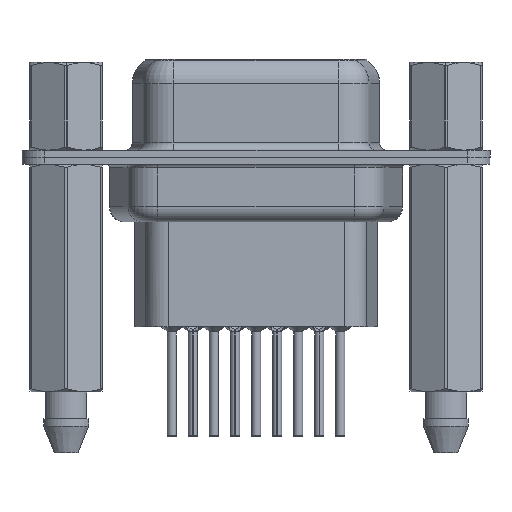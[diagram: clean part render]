
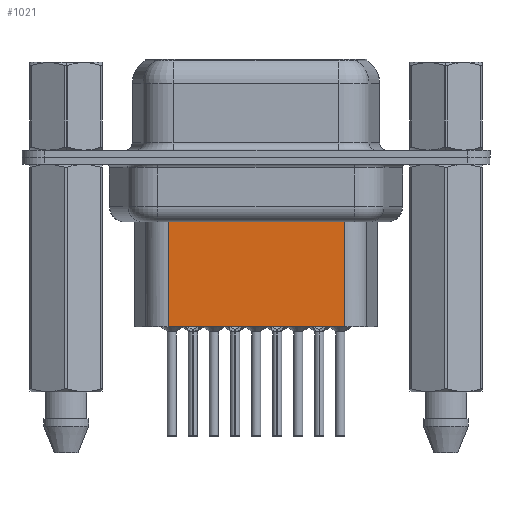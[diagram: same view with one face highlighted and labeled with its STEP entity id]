
A CAD part, front view. The second image highlights one B-rep face of the part: STEP entity #1021.
In plain terms, the highlighted planar face has unit normal (0, -1, 0).
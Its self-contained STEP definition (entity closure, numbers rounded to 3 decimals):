
#703 = ORIENTED_EDGE ( 'NONE', *, *, #12172, .T. ) ;
#1021 = ADVANCED_FACE ( 'NONE', ( #27451 ), #8354, .T. ) ;
#1368 = LINE ( 'NONE', #9865, #4313 ) ;
#1404 = DIRECTION ( 'NONE',  ( 1., 0., 0. ) ) ;
#1757 = DIRECTION ( 'NONE',  ( 0., 0., -1. ) ) ;
#2477 = CARTESIAN_POINT ( 'NONE',  ( 6.706, -3.5, -11.15 ) ) ;
#4313 = VECTOR ( 'NONE', #18347, 1000. ) ;
#4630 = VERTEX_POINT ( 'NONE', #13795 ) ;
#5192 = EDGE_CURVE ( 'NONE', #8631, #26141, #1368, .T. ) ;
#5831 = CARTESIAN_POINT ( 'NONE',  ( 6.706, -3.5, -3.1 ) ) ;
#6327 = EDGE_CURVE ( 'NONE', #8631, #4630, #18413, .T. ) ;
#6532 = VECTOR ( 'NONE', #9931, 1000. ) ;
#7393 = CARTESIAN_POINT ( 'NONE',  ( 18.294, -3.5, -11.15 ) ) ;
#8354 = PLANE ( 'NONE',  #12449 ) ;
#8631 = VERTEX_POINT ( 'NONE', #11443 ) ;
#9865 = CARTESIAN_POINT ( 'NONE',  ( 18.294, -3.5, -3.1 ) ) ;
#9931 = DIRECTION ( 'NONE',  ( -1., 0., 0. ) ) ;
#11034 = ORIENTED_EDGE ( 'NONE', *, *, #6327, .T. ) ;
#11443 = CARTESIAN_POINT ( 'NONE',  ( 18.294, -3.5, -4.097 ) ) ;
#11980 = VERTEX_POINT ( 'NONE', #21145 ) ;
#12172 = EDGE_CURVE ( 'NONE', #4630, #11980, #12220, .T. ) ;
#12220 = LINE ( 'NONE', #20705, #16073 ) ;
#12269 = ORIENTED_EDGE ( 'NONE', *, *, #21077, .F. ) ;
#12449 = AXIS2_PLACEMENT_3D ( 'NONE', #5831, #14080, #1404 ) ;
#13795 = CARTESIAN_POINT ( 'NONE',  ( 6.706, -3.5, -4.097 ) ) ;
#14080 = DIRECTION ( 'NONE',  ( 0., -1., 0. ) ) ;
#16073 = VECTOR ( 'NONE', #1757, 1000. ) ;
#18347 = DIRECTION ( 'NONE',  ( 0., 0., -1. ) ) ;
#18413 = LINE ( 'NONE', #26381, #6532 ) ;
#19394 = VECTOR ( 'NONE', #23533, 1000. ) ;
#20705 = CARTESIAN_POINT ( 'NONE',  ( 6.706, -3.5, -3.1 ) ) ;
#21077 = EDGE_CURVE ( 'NONE', #26141, #11980, #25773, .T. ) ;
#21145 = CARTESIAN_POINT ( 'NONE',  ( 6.706, -3.5, -11.15 ) ) ;
#23533 = DIRECTION ( 'NONE',  ( -1., 0., 0. ) ) ;
#23971 = ORIENTED_EDGE ( 'NONE', *, *, #5192, .F. ) ;
#25773 = LINE ( 'NONE', #2477, #19394 ) ;
#26141 = VERTEX_POINT ( 'NONE', #7393 ) ;
#26381 = CARTESIAN_POINT ( 'NONE',  ( 6.459, -3.5, -4.097 ) ) ;
#27238 = EDGE_LOOP ( 'NONE', ( #23971, #11034, #703, #12269 ) ) ;
#27451 = FACE_OUTER_BOUND ( 'NONE', #27238, .T. ) ;
